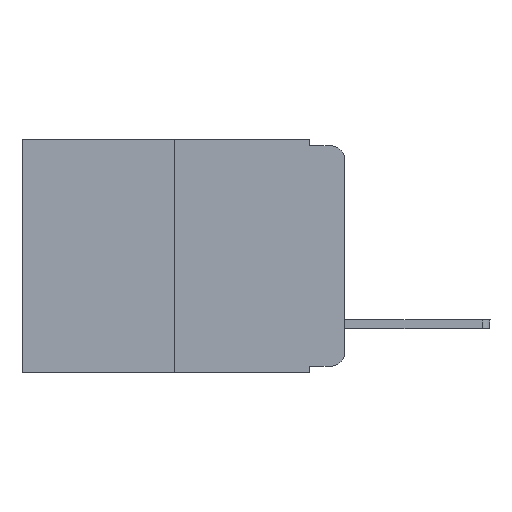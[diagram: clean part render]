
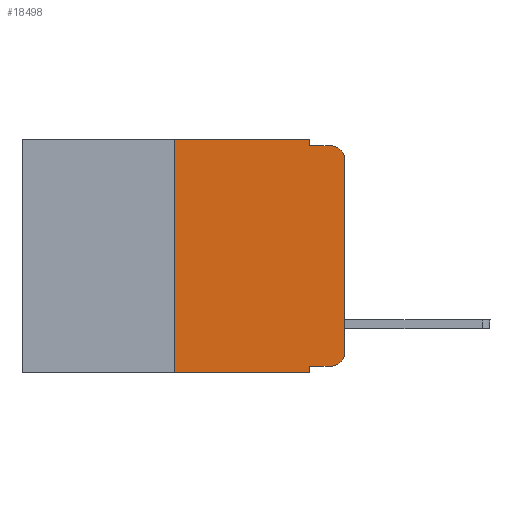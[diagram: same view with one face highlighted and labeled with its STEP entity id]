
A CAD part, left-side view. The second image highlights one B-rep face of the part: STEP entity #18498.
In plain terms, the highlighted planar face has unit normal (-1, 0, 0).
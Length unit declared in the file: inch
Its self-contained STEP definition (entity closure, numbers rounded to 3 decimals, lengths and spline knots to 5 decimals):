
#79 = EDGE_CURVE ( 'NONE', #11475, #13770, #18806, .T. ) ;
#457 = EDGE_CURVE ( 'NONE', #19345, #13705, #10892, .T. ) ;
#632 = EDGE_CURVE ( 'NONE', #13705, #1150, #11888, .T. ) ;
#813 = CARTESIAN_POINT ( 'NONE',  ( 0., 0.02, -0.313 ) ) ;
#829 = DIRECTION ( 'NONE',  ( 0., 0., -1. ) ) ;
#962 = VECTOR ( 'NONE', #5262, 39.37008 ) ;
#1150 = VERTEX_POINT ( 'NONE', #7054 ) ;
#1498 = CARTESIAN_POINT ( 'NONE',  ( 0., 0.051, -0.01 ) ) ;
#1776 = DIRECTION ( 'NONE',  ( 0., 0., -1. ) ) ;
#1984 = DIRECTION ( 'NONE',  ( 0., -1., 0. ) ) ;
#1987 = DIRECTION ( 'NONE',  ( 0., 0., -1. ) ) ;
#2032 = EDGE_CURVE ( 'NONE', #19345, #7892, #13240, .T. ) ;
#2099 = EDGE_CURVE ( 'NONE', #17623, #15768, #4329, .T. ) ;
#2310 = VECTOR ( 'NONE', #7751, 39.37008 ) ;
#2702 = ORIENTED_EDGE ( 'NONE', *, *, #3323, .F. ) ;
#2738 = AXIS2_PLACEMENT_3D ( 'NONE', #813, #6971, #1776 ) ;
#2791 = CARTESIAN_POINT ( 'NONE',  ( 0., 0.051, 0. ) ) ;
#3323 = EDGE_CURVE ( 'NONE', #15768, #8678, #18366, .T. ) ;
#4287 = CARTESIAN_POINT ( 'NONE',  ( 0., 0.051, 0. ) ) ;
#4329 = LINE ( 'NONE', #13343, #15891 ) ;
#5040 = EDGE_CURVE ( 'NONE', #1150, #15989, #16235, .T. ) ;
#5262 = DIRECTION ( 'NONE',  ( 0., 0., 1. ) ) ;
#5860 = DIRECTION ( 'NONE',  ( 0., 0., -1. ) ) ;
#6224 = EDGE_CURVE ( 'NONE', #17623, #7892, #15455, .T. ) ;
#6971 = DIRECTION ( 'NONE',  ( -1., 0., 0. ) ) ;
#7054 = CARTESIAN_POINT ( 'NONE',  ( 0., 0., -0.313 ) ) ;
#7179 = CARTESIAN_POINT ( 'NONE',  ( 0., 0., -0.03 ) ) ;
#7398 = EDGE_CURVE ( 'NONE', #8678, #11475, #18321, .T. ) ;
#7440 = AXIS2_PLACEMENT_3D ( 'NONE', #19300, #8236, #1987 ) ;
#7751 = DIRECTION ( 'NONE',  ( 0., -1., 0. ) ) ;
#7892 = VERTEX_POINT ( 'NONE', #15698 ) ;
#8236 = DIRECTION ( 'NONE',  ( 1., 0., 0. ) ) ;
#8668 = ORIENTED_EDGE ( 'NONE', *, *, #632, .T. ) ;
#8678 = VERTEX_POINT ( 'NONE', #19834 ) ;
#8739 = CARTESIAN_POINT ( 'NONE',  ( 0., 0.473, 0. ) ) ;
#9078 = CARTESIAN_POINT ( 'NONE',  ( 0., 0.051, -0.333 ) ) ;
#9129 = VECTOR ( 'NONE', #13449, 39.37008 ) ;
#9209 = CARTESIAN_POINT ( 'NONE',  ( 0., 0.473, -0.343 ) ) ;
#9608 = VECTOR ( 'NONE', #18778, 39.37008 ) ;
#9633 = ORIENTED_EDGE ( 'NONE', *, *, #7398, .F. ) ;
#9967 = CARTESIAN_POINT ( 'NONE',  ( 0., 0.02, -0.01 ) ) ;
#10012 = ORIENTED_EDGE ( 'NONE', *, *, #2099, .F. ) ;
#10165 = CARTESIAN_POINT ( 'NONE',  ( 0., 0.02, -0.333 ) ) ;
#10364 = CARTESIAN_POINT ( 'NONE',  ( 0., 0.02, -0.03 ) ) ;
#10453 = EDGE_LOOP ( 'NONE', ( #12299, #18576, #18375, #9633, #2702, #10012, #13009, #10571, #11546, #8668 ) ) ;
#10571 = ORIENTED_EDGE ( 'NONE', *, *, #2032, .F. ) ;
#10612 = VECTOR ( 'NONE', #5860, 39.37008 ) ;
#10892 = LINE ( 'NONE', #9078, #9608 ) ;
#11367 = CARTESIAN_POINT ( 'NONE',  ( 0., 0.25, -0.343 ) ) ;
#11475 = VERTEX_POINT ( 'NONE', #15027 ) ;
#11546 = ORIENTED_EDGE ( 'NONE', *, *, #457, .T. ) ;
#11888 = CIRCLE ( 'NONE', #2738, 0.02 ) ;
#12025 = EDGE_CURVE ( 'NONE', #15989, #13770, #13815, .T. ) ;
#12299 = ORIENTED_EDGE ( 'NONE', *, *, #5040, .T. ) ;
#13009 = ORIENTED_EDGE ( 'NONE', *, *, #6224, .T. ) ;
#13240 = LINE ( 'NONE', #2791, #10612 ) ;
#13343 = CARTESIAN_POINT ( 'NONE',  ( 0., 0.25, 0. ) ) ;
#13449 = DIRECTION ( 'NONE',  ( 0., -1., 0. ) ) ;
#13705 = VERTEX_POINT ( 'NONE', #10165 ) ;
#13770 = VERTEX_POINT ( 'NONE', #9967 ) ;
#13815 = CIRCLE ( 'NONE', #16115, 0.02 ) ;
#14059 = CARTESIAN_POINT ( 'NONE',  ( 0., 0.25, 0. ) ) ;
#14271 = VECTOR ( 'NONE', #1984, 39.37008 ) ;
#14880 = DIRECTION ( 'NONE',  ( -1., 0., 0. ) ) ;
#15027 = CARTESIAN_POINT ( 'NONE',  ( 0., 0.051, -0.01 ) ) ;
#15260 = DIRECTION ( 'NONE',  ( 0., 0., -1. ) ) ;
#15455 = LINE ( 'NONE', #9209, #14271 ) ;
#15698 = CARTESIAN_POINT ( 'NONE',  ( 0., 0.051, -0.343 ) ) ;
#15768 = VERTEX_POINT ( 'NONE', #14059 ) ;
#15832 = PLANE ( 'NONE',  #7440 ) ;
#15891 = VECTOR ( 'NONE', #17959, 39.37008 ) ;
#15958 = CARTESIAN_POINT ( 'NONE',  ( 0., 0.051, -0.333 ) ) ;
#15989 = VERTEX_POINT ( 'NONE', #7179 ) ;
#16115 = AXIS2_PLACEMENT_3D ( 'NONE', #10364, #14880, #829 ) ;
#16235 = LINE ( 'NONE', #19386, #962 ) ;
#16245 = VECTOR ( 'NONE', #15260, 39.37008 ) ;
#17623 = VERTEX_POINT ( 'NONE', #11367 ) ;
#17959 = DIRECTION ( 'NONE',  ( 0., 0., 1. ) ) ;
#18321 = LINE ( 'NONE', #4287, #16245 ) ;
#18366 = LINE ( 'NONE', #8739, #9129 ) ;
#18375 = ORIENTED_EDGE ( 'NONE', *, *, #79, .F. ) ;
#18498 = ADVANCED_FACE ( 'NONE', ( #19663 ), #15832, .F. ) ;
#18576 = ORIENTED_EDGE ( 'NONE', *, *, #12025, .T. ) ;
#18778 = DIRECTION ( 'NONE',  ( 0., -1., 0. ) ) ;
#18806 = LINE ( 'NONE', #1498, #2310 ) ;
#19300 = CARTESIAN_POINT ( 'NONE',  ( 0., 0.473, 0. ) ) ;
#19345 = VERTEX_POINT ( 'NONE', #15958 ) ;
#19386 = CARTESIAN_POINT ( 'NONE',  ( 0., 0., 0. ) ) ;
#19663 = FACE_OUTER_BOUND ( 'NONE', #10453, .T. ) ;
#19834 = CARTESIAN_POINT ( 'NONE',  ( 0., 0.051, 0. ) ) ;
